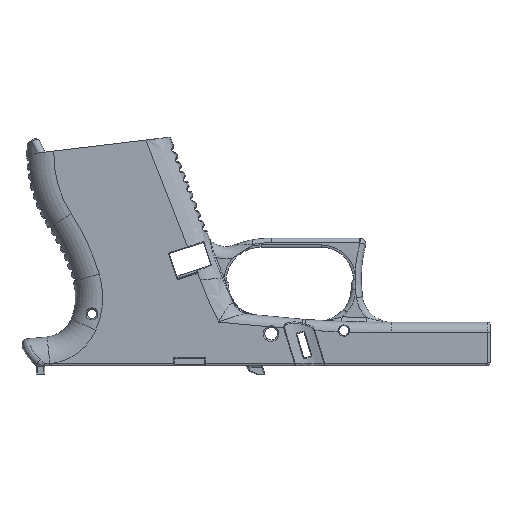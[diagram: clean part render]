
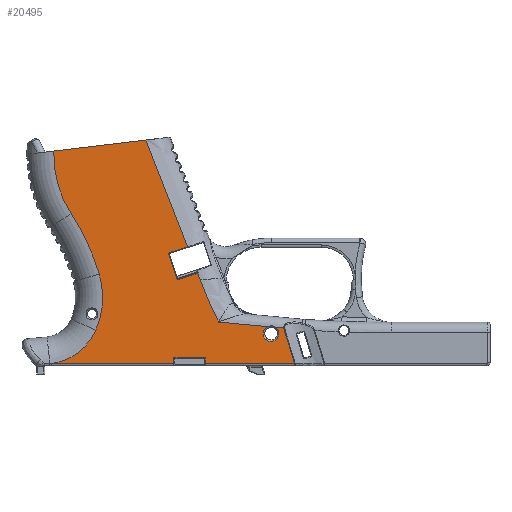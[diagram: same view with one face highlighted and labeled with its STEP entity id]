
A CAD part, front view. The second image highlights one B-rep face of the part: STEP entity #20495.
In plain terms, the highlighted planar face has unit normal (0, -1, 0).
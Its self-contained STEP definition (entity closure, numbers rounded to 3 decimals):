
#637=PLANE('',#22733);
#644=LINE('',#28511,#1657);
#722=LINE('',#29598,#1735);
#727=LINE('',#29612,#1740);
#730=LINE('',#29620,#1743);
#755=LINE('',#29925,#1768);
#756=LINE('',#29927,#1769);
#799=LINE('',#30519,#1812);
#832=LINE('',#31273,#1845);
#835=LINE('',#31653,#1848);
#837=LINE('',#31679,#1850);
#839=LINE('',#31687,#1852);
#1439=LINE('',#50382,#2452);
#1440=LINE('',#50383,#2453);
#1470=LINE('',#51210,#2483);
#1475=LINE('',#51246,#2488);
#1477=LINE('',#51284,#2490);
#1480=LINE('',#51292,#2493);
#1657=VECTOR('',#22788,10.);
#1735=VECTOR('',#22960,10.);
#1740=VECTOR('',#22973,10.);
#1743=VECTOR('',#22984,10.);
#1768=VECTOR('',#23039,10.);
#1769=VECTOR('',#23040,10.);
#1812=VECTOR('',#23297,10.);
#1845=VECTOR('',#23526,10.);
#1848=VECTOR('',#23577,10.);
#1850=VECTOR('',#23587,10.);
#1852=VECTOR('',#23595,10.);
#2452=VECTOR('',#27321,10.);
#2453=VECTOR('',#27322,10.);
#2483=VECTOR('',#27484,10.);
#2488=VECTOR('',#27507,10.);
#2490=VECTOR('',#27515,10.);
#2493=VECTOR('',#27524,10.);
#4780=FACE_OUTER_BOUND('',#6057,.T.);
#6057=EDGE_LOOP('',(#18974,#18975,#18976,#18977,#18978,#18979,#18980,#18981,
#18982,#18983,#18984,#18985,#18986,#18987,#18988,#18989,#18990,#18991,#18992,
#18993,#18994,#18995,#18996,#18997,#18998,#18999,#19000,#19001));
#6096=CIRCLE('',#20583,0.45);
#6098=CIRCLE('',#20587,0.45);
#6185=CIRCLE('',#20763,18.891);
#6233=CIRCLE('',#20829,77.599);
#6240=CIRCLE('',#20840,156.771);
#7109=CIRCLE('',#22404,2.625);
#7110=CIRCLE('',#22405,2.625);
#7141=CIRCLE('',#22473,0.8);
#7205=CIRCLE('',#22638,27.167);
#7231=CIRCLE('',#22734,35.645);
#7313=B_SPLINE_CURVE_WITH_KNOTS('',3,(#29637,#29638,#29639,#29640),
 .UNSPECIFIED.,.F.,.F.,(4,4),(-0.106,-0.092),
 .UNSPECIFIED.);
#7902=VERTEX_POINT('',#28491);
#7903=VERTEX_POINT('',#28510);
#8028=VERTEX_POINT('',#29500);
#8030=VERTEX_POINT('',#29527);
#8036=VERTEX_POINT('',#29595);
#8037=VERTEX_POINT('',#29597);
#8040=VERTEX_POINT('',#29605);
#8042=VERTEX_POINT('',#29610);
#8043=VERTEX_POINT('',#29616);
#8070=VERTEX_POINT('',#29926);
#8169=VERTEX_POINT('',#30516);
#8170=VERTEX_POINT('',#30518);
#8212=VERTEX_POINT('',#30891);
#8254=VERTEX_POINT('',#31271);
#8280=VERTEX_POINT('',#31631);
#8281=VERTEX_POINT('',#31633);
#8285=VERTEX_POINT('',#31650);
#8286=VERTEX_POINT('',#31652);
#8290=VERTEX_POINT('',#31677);
#8293=VERTEX_POINT('',#31685);
#8298=VERTEX_POINT('',#31736);
#9513=VERTEX_POINT('',#50370);
#9514=VERTEX_POINT('',#50371);
#9515=VERTEX_POINT('',#50385);
#9563=VERTEX_POINT('',#51208);
#9567=VERTEX_POINT('',#51222);
#9569=VERTEX_POINT('',#51243);
#9572=VERTEX_POINT('',#51281);
#9764=EDGE_CURVE('',#7902,#7903,#644,.T.);
#9940=EDGE_CURVE('',#8036,#8037,#722,.T.);
#9945=EDGE_CURVE('',#8040,#8036,#6096,.T.);
#9947=EDGE_CURVE('',#8042,#8040,#727,.T.);
#9951=EDGE_CURVE('',#8043,#8042,#6098,.T.);
#9952=EDGE_CURVE('',#8028,#8043,#730,.T.);
#9953=EDGE_CURVE('',#8037,#8030,#7313,.T.);
#9998=EDGE_CURVE('',#8028,#7903,#755,.T.);
#9999=EDGE_CURVE('',#8070,#8030,#756,.T.);
#10134=EDGE_CURVE('',#8169,#8170,#799,.T.);
#10204=EDGE_CURVE('',#8170,#8212,#6185,.T.);
#10266=EDGE_CURVE('',#8254,#8169,#832,.T.);
#10293=EDGE_CURVE('',#8280,#8281,#6233,.T.);
#10298=EDGE_CURVE('',#8285,#8286,#835,.T.);
#10304=EDGE_CURVE('',#8290,#8285,#837,.T.);
#10308=EDGE_CURVE('',#8293,#8290,#839,.T.);
#10313=EDGE_CURVE('',#8070,#8298,#6240,.T.);
#12401=EDGE_CURVE('',#9513,#8293,#1439,.T.);
#12402=EDGE_CURVE('',#8298,#9514,#1440,.T.);
#12403=EDGE_CURVE('',#9514,#9515,#7109,.T.);
#12405=EDGE_CURVE('',#9515,#9513,#7110,.T.);
#12496=EDGE_CURVE('',#8286,#9563,#1470,.T.);
#12503=EDGE_CURVE('',#9567,#8254,#7141,.T.);
#12507=EDGE_CURVE('',#9569,#9567,#1475,.T.);
#12512=EDGE_CURVE('',#9572,#9569,#1477,.T.);
#12517=EDGE_CURVE('',#9563,#9572,#1480,.T.);
#12742=EDGE_CURVE('',#8212,#8280,#7205,.T.);
#12866=EDGE_CURVE('',#8281,#7902,#7231,.T.);
#18974=ORIENTED_EDGE('',*,*,#10304,.F.);
#18975=ORIENTED_EDGE('',*,*,#10308,.F.);
#18976=ORIENTED_EDGE('',*,*,#12401,.F.);
#18977=ORIENTED_EDGE('',*,*,#12405,.F.);
#18978=ORIENTED_EDGE('',*,*,#12403,.F.);
#18979=ORIENTED_EDGE('',*,*,#12402,.F.);
#18980=ORIENTED_EDGE('',*,*,#10313,.F.);
#18981=ORIENTED_EDGE('',*,*,#9999,.T.);
#18982=ORIENTED_EDGE('',*,*,#9953,.F.);
#18983=ORIENTED_EDGE('',*,*,#9940,.F.);
#18984=ORIENTED_EDGE('',*,*,#9945,.F.);
#18985=ORIENTED_EDGE('',*,*,#9947,.F.);
#18986=ORIENTED_EDGE('',*,*,#9951,.F.);
#18987=ORIENTED_EDGE('',*,*,#9952,.F.);
#18988=ORIENTED_EDGE('',*,*,#9998,.T.);
#18989=ORIENTED_EDGE('',*,*,#9764,.F.);
#18990=ORIENTED_EDGE('',*,*,#12866,.F.);
#18991=ORIENTED_EDGE('',*,*,#10293,.F.);
#18992=ORIENTED_EDGE('',*,*,#12742,.F.);
#18993=ORIENTED_EDGE('',*,*,#10204,.F.);
#18994=ORIENTED_EDGE('',*,*,#10134,.F.);
#18995=ORIENTED_EDGE('',*,*,#10266,.F.);
#18996=ORIENTED_EDGE('',*,*,#12503,.F.);
#18997=ORIENTED_EDGE('',*,*,#12507,.F.);
#18998=ORIENTED_EDGE('',*,*,#12512,.F.);
#18999=ORIENTED_EDGE('',*,*,#12517,.F.);
#19000=ORIENTED_EDGE('',*,*,#12496,.F.);
#19001=ORIENTED_EDGE('',*,*,#10298,.F.);
#20495=ADVANCED_FACE('',(#4780),#637,.F.);
#20583=AXIS2_PLACEMENT_3D('',#29607,#22968,#22969);
#20587=AXIS2_PLACEMENT_3D('',#29618,#22980,#22981);
#20763=AXIS2_PLACEMENT_3D('',#30892,#23417,#23418);
#20829=AXIS2_PLACEMENT_3D('',#31634,#23568,#23569);
#20840=AXIS2_PLACEMENT_3D('',#31737,#23598,#23599);
#22404=AXIS2_PLACEMENT_3D('',#50386,#27325,#27326);
#22405=AXIS2_PLACEMENT_3D('',#50388,#27328,#27329);
#22473=AXIS2_PLACEMENT_3D('',#51229,#27497,#27498);
#22638=AXIS2_PLACEMENT_3D('',#53190,#27935,#27936);
#22733=AXIS2_PLACEMENT_3D('',#54009,#28193,#28194);
#22734=AXIS2_PLACEMENT_3D('',#54010,#28195,#28196);
#22788=DIRECTION('',(0.993,0.,0.119));
#22960=DIRECTION('',(0.951,0.,0.309));
#22968=DIRECTION('center_axis',(0.,-1.,0.));
#22969=DIRECTION('ref_axis',(-0.454,0.,-0.891));
#22973=DIRECTION('',(0.309,0.,-0.951));
#22980=DIRECTION('center_axis',(0.,-1.,0.));
#22981=DIRECTION('ref_axis',(-0.891,0.,0.454));
#22984=DIRECTION('',(-0.951,0.,-0.309));
#23039=DIRECTION('',(-0.363,0.,0.932));
#23040=DIRECTION('',(-0.363,0.,0.932));
#23297=DIRECTION('',(-1.,0.,0.));
#23417=DIRECTION('center_axis',(0.,-1.,0.));
#23418=DIRECTION('ref_axis',(0.592,0.,-0.806));
#23526=DIRECTION('',(0.,0.,-1.));
#23568=DIRECTION('center_axis',(0.,-1.,0.));
#23569=DIRECTION('ref_axis',(0.907,0.,0.421));
#23577=DIRECTION('',(0.,0.,1.));
#23587=DIRECTION('',(-1.,0.,0.));
#23595=DIRECTION('',(0.292,0.,-0.956));
#23598=DIRECTION('center_axis',(0.,-1.,0.));
#23599=DIRECTION('ref_axis',(-0.937,0.,-0.35));
#27321=DIRECTION('',(0.996,0.,-0.092));
#27322=DIRECTION('',(0.996,0.,-0.092));
#27325=DIRECTION('center_axis',(0.,-1.,0.));
#27326=DIRECTION('ref_axis',(-1.,0.,0.));
#27328=DIRECTION('center_axis',(0.,-1.,0.));
#27329=DIRECTION('ref_axis',(-1.,0.,0.));
#27484=DIRECTION('',(-1.,0.,0.));
#27497=DIRECTION('center_axis',(0.,-1.,0.));
#27498=DIRECTION('ref_axis',(-0.707,0.,0.707));
#27507=DIRECTION('',(0.,0.,-1.));
#27515=DIRECTION('',(-1.,0.,0.));
#27524=DIRECTION('',(0.,0.,1.));
#27935=DIRECTION('center_axis',(0.,-1.,0.));
#27936=DIRECTION('ref_axis',(0.998,0.,-0.06));
#28193=DIRECTION('center_axis',(0.,1.,0.));
#28194=DIRECTION('ref_axis',(1.,0.,0.));
#28195=DIRECTION('center_axis',(0.,1.,0.));
#28196=DIRECTION('ref_axis',(-0.961,0.,-0.276));
#28491=CARTESIAN_POINT('',(-68.982,-11.5,45.003));
#28510=CARTESIAN_POINT('',(-38.322,-11.5,48.672));
#28511=CARTESIAN_POINT('',(-6.737,-11.5,52.452));
#29500=CARTESIAN_POINT('',(-24.467,-11.5,13.103));
#29527=CARTESIAN_POINT('',(-21.075,-11.5,4.396));
#29595=CARTESIAN_POINT('',(-27.466,-11.5,2.245));
#29597=CARTESIAN_POINT('',(-21.284,-11.5,4.253));
#29598=CARTESIAN_POINT('',(-11.372,-11.5,7.474));
#29605=CARTESIAN_POINT('',(-28.033,-11.5,2.534));
#29607=CARTESIAN_POINT('Origin',(-27.605,-11.5,2.673));
#29610=CARTESIAN_POINT('',(-30.659,-11.5,10.618));
#29612=CARTESIAN_POINT('',(-28.119,-11.5,2.799));
#29616=CARTESIAN_POINT('',(-30.37,-11.5,11.185));
#29618=CARTESIAN_POINT('Origin',(-30.231,-11.5,10.757));
#29620=CARTESIAN_POINT('',(-17.605,-11.5,15.332));
#29637=CARTESIAN_POINT('Ctrl Pts',(-21.284,-11.5,4.253));
#29638=CARTESIAN_POINT('Ctrl Pts',(-21.203,-11.5,4.28));
#29639=CARTESIAN_POINT('Ctrl Pts',(-21.129,-11.5,4.33));
#29640=CARTESIAN_POINT('Ctrl Pts',(-21.075,-11.5,4.396));
#29925=CARTESIAN_POINT('',(-37.545,-11.5,46.678));
#29926=CARTESIAN_POINT('',(-20.166,-11.5,2.06));
#29927=CARTESIAN_POINT('',(-37.545,-11.5,46.678));
#30516=CARTESIAN_POINT('',(-29.05,-11.5,-25.75));
#30518=CARTESIAN_POINT('',(-69.695,-11.5,-25.75));
#30519=CARTESIAN_POINT('',(37.236,-11.5,-25.75));
#30891=CARTESIAN_POINT('',(-55.002,-11.5,-14.602));
#30892=CARTESIAN_POINT('Origin',(-72.315,-11.5,-7.041));
#31271=CARTESIAN_POINT('',(-29.05,-11.5,-25.475));
#31273=CARTESIAN_POINT('',(-29.05,-11.5,-7.056));
#31631=CARTESIAN_POINT('',(-53.881,-11.5,4.09));
#31633=CARTESIAN_POINT('',(-63.213,-11.5,24.169));
#31634=CARTESIAN_POINT('Origin',(-128.196,-11.5,-18.243));
#31650=CARTESIAN_POINT('',(-18.45,-11.5,-25.75));
#31652=CARTESIAN_POINT('',(-18.45,-11.5,-24.675));
#31653=CARTESIAN_POINT('',(-18.45,-11.5,-7.818));
#31677=CARTESIAN_POINT('',(11.185,-11.5,-25.75));
#31679=CARTESIAN_POINT('',(37.236,-11.5,-25.75));
#31685=CARTESIAN_POINT('',(7.57,-11.5,-13.924));
#31687=CARTESIAN_POINT('',(5.553,-11.5,-7.328));
#31736=CARTESIAN_POINT('',(-14.141,-11.5,-11.929));
#31737=CARTESIAN_POINT('Origin',(126.663,-11.5,57.001));
#50370=CARTESIAN_POINT('',(4.906,-11.5,-13.679));
#50371=CARTESIAN_POINT('',(2.19,-11.5,-13.43));
#50382=CARTESIAN_POINT('',(4.861,-11.5,-13.675));
#50383=CARTESIAN_POINT('',(4.861,-11.5,-13.675));
#50385=CARTESIAN_POINT('',(5.968,-11.5,-15.788));
#50386=CARTESIAN_POINT('Origin',(3.343,-11.5,-15.788));
#50388=CARTESIAN_POINT('Origin',(3.343,-11.5,-15.788));
#51208=CARTESIAN_POINT('',(-18.52,-11.5,-24.675));
#51210=CARTESIAN_POINT('',(-10.264,-11.5,-24.675));
#51222=CARTESIAN_POINT('',(-28.98,-11.5,-25.148));
#51229=CARTESIAN_POINT('Origin',(-28.25,-11.5,-25.475));
#51243=CARTESIAN_POINT('',(-28.98,-11.5,-23.745));
#51246=CARTESIAN_POINT('',(-28.98,-11.5,-7.056));
#51281=CARTESIAN_POINT('',(-18.52,-11.5,-23.745));
#51284=CARTESIAN_POINT('',(-10.264,-11.5,-23.745));
#51292=CARTESIAN_POINT('',(-18.52,-11.5,-7.056));
#53190=CARTESIAN_POINT('Origin',(-79.899,-11.5,-3.729));
#54009=CARTESIAN_POINT('Origin',(-1.777,-11.5,10.863));
#54010=CARTESIAN_POINT('Origin',(-33.363,-11.5,43.651));
